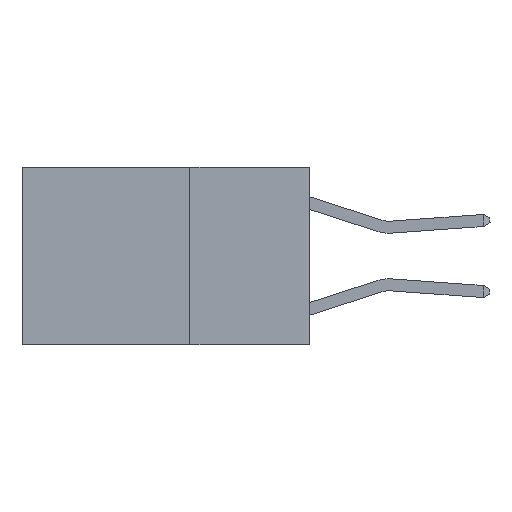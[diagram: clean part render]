
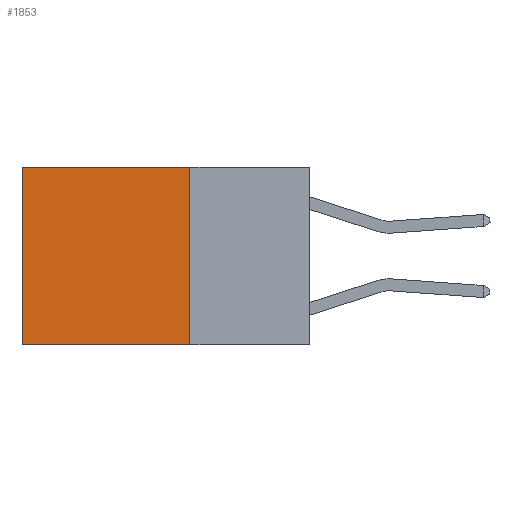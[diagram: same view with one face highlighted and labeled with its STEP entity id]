
A CAD part, left-side view. The second image highlights one B-rep face of the part: STEP entity #1853.
In plain terms, the highlighted planar face has unit normal (-1, 0, 0).
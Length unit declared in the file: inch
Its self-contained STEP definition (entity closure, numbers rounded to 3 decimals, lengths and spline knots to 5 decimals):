
#234 = CARTESIAN_POINT ( 'NONE',  ( 0.2625, 0.25, -0.37 ) ) ;
#601 = VECTOR ( 'NONE', #7983, 39.37008 ) ;
#1035 = VERTEX_POINT ( 'NONE', #12371 ) ;
#1416 = ORIENTED_EDGE ( 'NONE', *, *, #15844, .F. ) ;
#1463 = DIRECTION ( 'NONE',  ( 0., 0., -1. ) ) ;
#1853 = ADVANCED_FACE ( 'NONE', ( #3829 ), #12949, .F. ) ;
#2231 = ORIENTED_EDGE ( 'NONE', *, *, #3783, .F. ) ;
#2269 = LINE ( 'NONE', #12782, #8297 ) ;
#2760 = AXIS2_PLACEMENT_3D ( 'NONE', #5185, #6635, #9034 ) ;
#3783 = EDGE_CURVE ( 'NONE', #3840, #6119, #5761, .T. ) ;
#3829 = FACE_OUTER_BOUND ( 'NONE', #11758, .T. ) ;
#3840 = VERTEX_POINT ( 'NONE', #16383 ) ;
#4692 = CARTESIAN_POINT ( 'NONE',  ( 0.2625, 0.6, -0.37 ) ) ;
#5185 = CARTESIAN_POINT ( 'NONE',  ( 0.2625, 0.25, 0. ) ) ;
#5761 = LINE ( 'NONE', #9271, #601 ) ;
#6119 = VERTEX_POINT ( 'NONE', #7124 ) ;
#6623 = EDGE_CURVE ( 'NONE', #3840, #1035, #2269, .T. ) ;
#6635 = DIRECTION ( 'NONE',  ( 1., 0., 0. ) ) ;
#7124 = CARTESIAN_POINT ( 'NONE',  ( 0.2625, 0.25, -0.37 ) ) ;
#7129 = EDGE_CURVE ( 'NONE', #1035, #8079, #7894, .T. ) ;
#7894 = LINE ( 'NONE', #11870, #14964 ) ;
#7983 = DIRECTION ( 'NONE',  ( 0., 0., -1. ) ) ;
#8079 = VERTEX_POINT ( 'NONE', #4692 ) ;
#8297 = VECTOR ( 'NONE', #16759, 39.37008 ) ;
#9034 = DIRECTION ( 'NONE',  ( 0., 0., -1. ) ) ;
#9271 = CARTESIAN_POINT ( 'NONE',  ( 0.2625, 0.25, 0. ) ) ;
#9891 = ORIENTED_EDGE ( 'NONE', *, *, #6623, .T. ) ;
#11758 = EDGE_LOOP ( 'NONE', ( #14505, #1416, #2231, #9891 ) ) ;
#11870 = CARTESIAN_POINT ( 'NONE',  ( 0.2625, 0.6, 0. ) ) ;
#12371 = CARTESIAN_POINT ( 'NONE',  ( 0.2625, 0.6, 0. ) ) ;
#12782 = CARTESIAN_POINT ( 'NONE',  ( 0.2625, 0.25, 0. ) ) ;
#12949 = PLANE ( 'NONE',  #2760 ) ;
#13371 = LINE ( 'NONE', #234, #16075 ) ;
#14505 = ORIENTED_EDGE ( 'NONE', *, *, #7129, .T. ) ;
#14853 = DIRECTION ( 'NONE',  ( 0., 1., 0. ) ) ;
#14964 = VECTOR ( 'NONE', #1463, 39.37008 ) ;
#15844 = EDGE_CURVE ( 'NONE', #6119, #8079, #13371, .T. ) ;
#16075 = VECTOR ( 'NONE', #14853, 39.37008 ) ;
#16383 = CARTESIAN_POINT ( 'NONE',  ( 0.2625, 0.25, 0. ) ) ;
#16759 = DIRECTION ( 'NONE',  ( 0., 1., 0. ) ) ;
